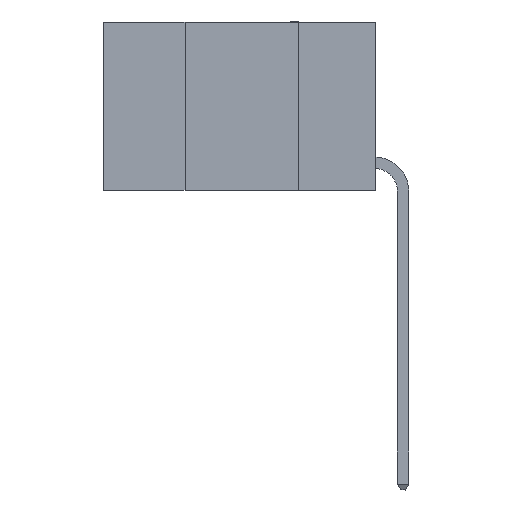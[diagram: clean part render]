
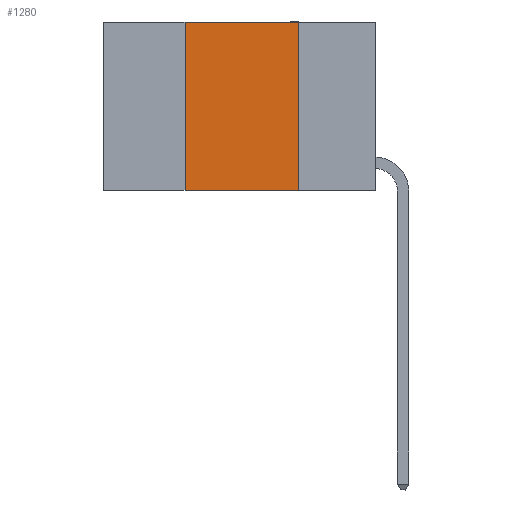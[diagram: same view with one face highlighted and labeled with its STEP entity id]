
A CAD part, left-side view. The second image highlights one B-rep face of the part: STEP entity #1280.
In plain terms, the highlighted planar face has unit normal (-1, 0, 0).
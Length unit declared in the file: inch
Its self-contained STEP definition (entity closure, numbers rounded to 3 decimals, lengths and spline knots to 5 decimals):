
#1278 = LINE ( 'NONE', #7943, #14317 ) ;
#1280 = ADVANCED_FACE ( 'NONE', ( #15833 ), #7413, .F. ) ;
#1380 = AXIS2_PLACEMENT_3D ( 'NONE', #17080, #24593, #13249 ) ;
#3703 = VERTEX_POINT ( 'NONE', #11118 ) ;
#4055 = EDGE_CURVE ( 'NONE', #5402, #6622, #11048, .T. ) ;
#5296 = VECTOR ( 'NONE', #23433, 39.37008 ) ;
#5402 = VERTEX_POINT ( 'NONE', #16077 ) ;
#6622 = VERTEX_POINT ( 'NONE', #12313 ) ;
#7413 = PLANE ( 'NONE',  #1380 ) ;
#7943 = CARTESIAN_POINT ( 'NONE',  ( 0., 0.42, 0. ) ) ;
#9412 = EDGE_CURVE ( 'NONE', #3703, #13310, #18247, .T. ) ;
#9907 = DIRECTION ( 'NONE',  ( 0., 0., 1. ) ) ;
#10829 = CARTESIAN_POINT ( 'NONE',  ( 0., 0.6, 0. ) ) ;
#11048 = LINE ( 'NONE', #15926, #5296 ) ;
#11118 = CARTESIAN_POINT ( 'NONE',  ( 0., 0.42, 0. ) ) ;
#11394 = ORIENTED_EDGE ( 'NONE', *, *, #9412, .F. ) ;
#12078 = EDGE_CURVE ( 'NONE', #13310, #6622, #22487, .T. ) ;
#12313 = CARTESIAN_POINT ( 'NONE',  ( 0., 0.17, -0.37 ) ) ;
#12782 = DIRECTION ( 'NONE',  ( 0., -1., 0. ) ) ;
#13189 = CARTESIAN_POINT ( 'NONE',  ( 0., 0.17, 0. ) ) ;
#13249 = DIRECTION ( 'NONE',  ( 0., 0., -1. ) ) ;
#13310 = VERTEX_POINT ( 'NONE', #20943 ) ;
#13717 = ORIENTED_EDGE ( 'NONE', *, *, #19906, .F. ) ;
#14317 = VECTOR ( 'NONE', #9907, 39.37008 ) ;
#14486 = ORIENTED_EDGE ( 'NONE', *, *, #12078, .F. ) ;
#15833 = FACE_OUTER_BOUND ( 'NONE', #16871, .T. ) ;
#15926 = CARTESIAN_POINT ( 'NONE',  ( 0., 0.6, -0.37 ) ) ;
#16077 = CARTESIAN_POINT ( 'NONE',  ( 0., 0.42, -0.37 ) ) ;
#16871 = EDGE_LOOP ( 'NONE', ( #14486, #11394, #13717, #22894 ) ) ;
#17080 = CARTESIAN_POINT ( 'NONE',  ( 0., 0.6, 0. ) ) ;
#17530 = VECTOR ( 'NONE', #20869, 39.37008 ) ;
#18247 = LINE ( 'NONE', #10829, #22628 ) ;
#19906 = EDGE_CURVE ( 'NONE', #5402, #3703, #1278, .T. ) ;
#20869 = DIRECTION ( 'NONE',  ( 0., 0., -1. ) ) ;
#20943 = CARTESIAN_POINT ( 'NONE',  ( 0., 0.17, 0. ) ) ;
#22487 = LINE ( 'NONE', #13189, #17530 ) ;
#22628 = VECTOR ( 'NONE', #12782, 39.37008 ) ;
#22894 = ORIENTED_EDGE ( 'NONE', *, *, #4055, .T. ) ;
#23433 = DIRECTION ( 'NONE',  ( 0., -1., 0. ) ) ;
#24593 = DIRECTION ( 'NONE',  ( 1., 0., 0. ) ) ;
